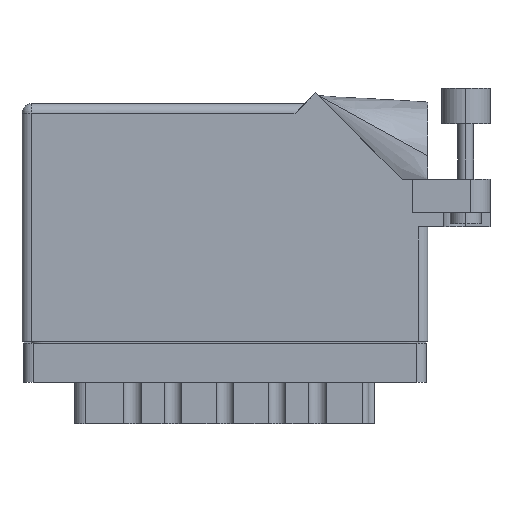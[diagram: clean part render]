
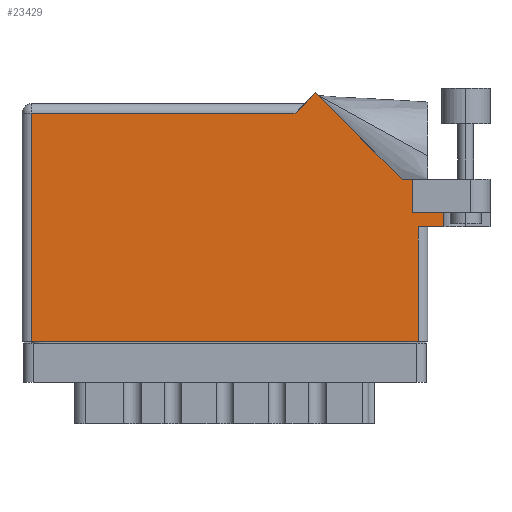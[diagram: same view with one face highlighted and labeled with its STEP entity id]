
A CAD part, front view. The second image highlights one B-rep face of the part: STEP entity #23429.
In plain terms, the highlighted face is planar.
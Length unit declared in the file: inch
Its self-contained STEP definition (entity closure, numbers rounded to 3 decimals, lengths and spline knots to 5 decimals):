
#731 = CARTESIAN_POINT ( 'NONE',  ( 0.062, 0., 0. ) ) ;
#956 = VECTOR ( 'NONE', #18990, 39.37008 ) ;
#1591 = VECTOR ( 'NONE', #9418, 39.37008 ) ;
#2251 = VERTEX_POINT ( 'NONE', #19079 ) ;
#3348 = ORIENTED_EDGE ( 'NONE', *, *, #6374, .T. ) ;
#4837 = VECTOR ( 'NONE', #8900, 39.37008 ) ;
#5656 = VERTEX_POINT ( 'NONE', #32921 ) ;
#5841 = ORIENTED_EDGE ( 'NONE', *, *, #21255, .T. ) ;
#6374 = EDGE_CURVE ( 'NONE', #49694, #14060, #45282, .T. ) ;
#6771 = CARTESIAN_POINT ( 'NONE',  ( 0., 1.53, 0. ) ) ;
#7487 = CARTESIAN_POINT ( 'NONE',  ( 2.612, 0.737, 0. ) ) ;
#8549 = VECTOR ( 'NONE', #8611, 39.37008 ) ;
#8611 = DIRECTION ( 'NONE',  ( -0.707, 0.707, 0. ) ) ;
#8688 = CARTESIAN_POINT ( 'NONE',  ( 2.44642, 1.044, 0. ) ) ;
#8805 = CARTESIAN_POINT ( 'NONE',  ( 2.7135, 1.16177, 0. ) ) ;
#8900 = DIRECTION ( 'NONE',  ( -1., 0., 0. ) ) ;
#9418 = DIRECTION ( 'NONE',  ( 1., 0., 0. ) ) ;
#9726 = ORIENTED_EDGE ( 'NONE', *, *, #26454, .F. ) ;
#9924 = ORIENTED_EDGE ( 'NONE', *, *, #41849, .T. ) ;
#10899 = CARTESIAN_POINT ( 'NONE',  ( 1.88971, 1.60071, 0. ) ) ;
#11062 = CARTESIAN_POINT ( 'NONE',  ( 0., 0., 0. ) ) ;
#11097 = VECTOR ( 'NONE', #14930, 39.37008 ) ;
#11523 = CARTESIAN_POINT ( 'NONE',  ( 2.512, 1.044, 0. ) ) ;
#11667 = CARTESIAN_POINT ( 'NONE',  ( 1.757, 1.468, 0. ) ) ;
#12048 = AXIS2_PLACEMENT_3D ( 'NONE', #6771, #48968, #30167 ) ;
#13463 = EDGE_CURVE ( 'NONE', #2251, #13603, #46112, .T. ) ;
#13601 = ORIENTED_EDGE ( 'NONE', *, *, #29436, .T. ) ;
#13603 = VERTEX_POINT ( 'NONE', #20125 ) ;
#14060 = VERTEX_POINT ( 'NONE', #10899 ) ;
#14112 = DIRECTION ( 'NONE',  ( 0., -1., 0. ) ) ;
#14684 = VERTEX_POINT ( 'NONE', #11667 ) ;
#14930 = DIRECTION ( 'NONE',  ( 1., 0., 0. ) ) ;
#15152 = CARTESIAN_POINT ( 'NONE',  ( 2.55, 0.737, 0. ) ) ;
#15623 = ORIENTED_EDGE ( 'NONE', *, *, #35452, .F. ) ;
#15878 = DIRECTION ( 'NONE',  ( 1., 0., 0. ) ) ;
#16529 = DIRECTION ( 'NONE',  ( 0., -1., 0. ) ) ;
#18141 = ORIENTED_EDGE ( 'NONE', *, *, #30896, .T. ) ;
#18347 = DIRECTION ( 'NONE',  ( -0.707, -0.707, 0. ) ) ;
#18990 = DIRECTION ( 'NONE',  ( 0., 1., 0. ) ) ;
#19055 = DIRECTION ( 'NONE',  ( -1., 0., 0. ) ) ;
#19079 = CARTESIAN_POINT ( 'NONE',  ( 2.55, 0., 0. ) ) ;
#20125 = CARTESIAN_POINT ( 'NONE',  ( 2.55, 0.737, 0. ) ) ;
#20441 = VERTEX_POINT ( 'NONE', #42067 ) ;
#21255 = EDGE_CURVE ( 'NONE', #39531, #49694, #41624, .T. ) ;
#21260 = CARTESIAN_POINT ( 'NONE',  ( 2.7135, 0.831, 0. ) ) ;
#22270 = EDGE_CURVE ( 'NONE', #34037, #47778, #24036, .T. ) ;
#22833 = LINE ( 'NONE', #36147, #4837 ) ;
#23429 = ADVANCED_FACE ( 'NONE', ( #29396 ), #44976, .F. ) ;
#23606 = DIRECTION ( 'NONE',  ( 0., 1., 0. ) ) ;
#23881 = CARTESIAN_POINT ( 'NONE',  ( 2.44642, 1.044, 0. ) ) ;
#24036 = LINE ( 'NONE', #45091, #46343 ) ;
#24296 = ORIENTED_EDGE ( 'NONE', *, *, #47212, .T. ) ;
#26454 = EDGE_CURVE ( 'NONE', #39214, #5656, #48173, .T. ) ;
#26705 = EDGE_CURVE ( 'NONE', #14060, #14684, #36182, .T. ) ;
#28435 = LINE ( 'NONE', #35591, #38064 ) ;
#29396 = FACE_OUTER_BOUND ( 'NONE', #39062, .T. ) ;
#29436 = EDGE_CURVE ( 'NONE', #13603, #5656, #32277, .T. ) ;
#30167 = DIRECTION ( 'NONE',  ( -1., 0., 0. ) ) ;
#30896 = EDGE_CURVE ( 'NONE', #47778, #2251, #37582, .T. ) ;
#31075 = ORIENTED_EDGE ( 'NONE', *, *, #13463, .T. ) ;
#32046 = VECTOR ( 'NONE', #19055, 39.37008 ) ;
#32277 = LINE ( 'NONE', #7487, #43068 ) ;
#32921 = CARTESIAN_POINT ( 'NONE',  ( 2.7135, 0.737, 0. ) ) ;
#34037 = VERTEX_POINT ( 'NONE', #49382 ) ;
#34964 = VECTOR ( 'NONE', #16529, 39.37008 ) ;
#35452 = EDGE_CURVE ( 'NONE', #20441, #39214, #44983, .T. ) ;
#35591 = CARTESIAN_POINT ( 'NONE',  ( 2.512, 0.831, 0. ) ) ;
#36009 = CARTESIAN_POINT ( 'NONE',  ( 2.512, 0.831, 0. ) ) ;
#36147 = CARTESIAN_POINT ( 'NONE',  ( 0., 1.468, 0. ) ) ;
#36182 = LINE ( 'NONE', #44615, #45214 ) ;
#37582 = LINE ( 'NONE', #11062, #11097 ) ;
#38064 = VECTOR ( 'NONE', #23606, 39.37008 ) ;
#39062 = EDGE_LOOP ( 'NONE', ( #18141, #31075, #13601, #9726, #15623, #9924, #5841, #3348, #45461, #24296, #41667 ) ) ;
#39214 = VERTEX_POINT ( 'NONE', #21260 ) ;
#39531 = VERTEX_POINT ( 'NONE', #11523 ) ;
#41624 = LINE ( 'NONE', #42769, #32046 ) ;
#41667 = ORIENTED_EDGE ( 'NONE', *, *, #22270, .T. ) ;
#41849 = EDGE_CURVE ( 'NONE', #20441, #39531, #28435, .T. ) ;
#42067 = CARTESIAN_POINT ( 'NONE',  ( 2.512, 0.831, 0. ) ) ;
#42769 = CARTESIAN_POINT ( 'NONE',  ( 3.012, 1.044, 0. ) ) ;
#43068 = VECTOR ( 'NONE', #15878, 39.37008 ) ;
#44615 = CARTESIAN_POINT ( 'NONE',  ( 1.819, 1.53, 0. ) ) ;
#44976 = PLANE ( 'NONE',  #12048 ) ;
#44983 = LINE ( 'NONE', #36009, #1591 ) ;
#45091 = CARTESIAN_POINT ( 'NONE',  ( 0.062, 0., 0. ) ) ;
#45214 = VECTOR ( 'NONE', #18347, 39.37008 ) ;
#45282 = LINE ( 'NONE', #23881, #8549 ) ;
#45461 = ORIENTED_EDGE ( 'NONE', *, *, #26705, .T. ) ;
#46112 = LINE ( 'NONE', #15152, #956 ) ;
#46343 = VECTOR ( 'NONE', #14112, 39.37008 ) ;
#47212 = EDGE_CURVE ( 'NONE', #14684, #34037, #22833, .T. ) ;
#47778 = VERTEX_POINT ( 'NONE', #731 ) ;
#48173 = LINE ( 'NONE', #8805, #34964 ) ;
#48968 = DIRECTION ( 'NONE',  ( 0., 0., -1. ) ) ;
#49382 = CARTESIAN_POINT ( 'NONE',  ( 0.062, 1.468, 0. ) ) ;
#49694 = VERTEX_POINT ( 'NONE', #8688 ) ;
